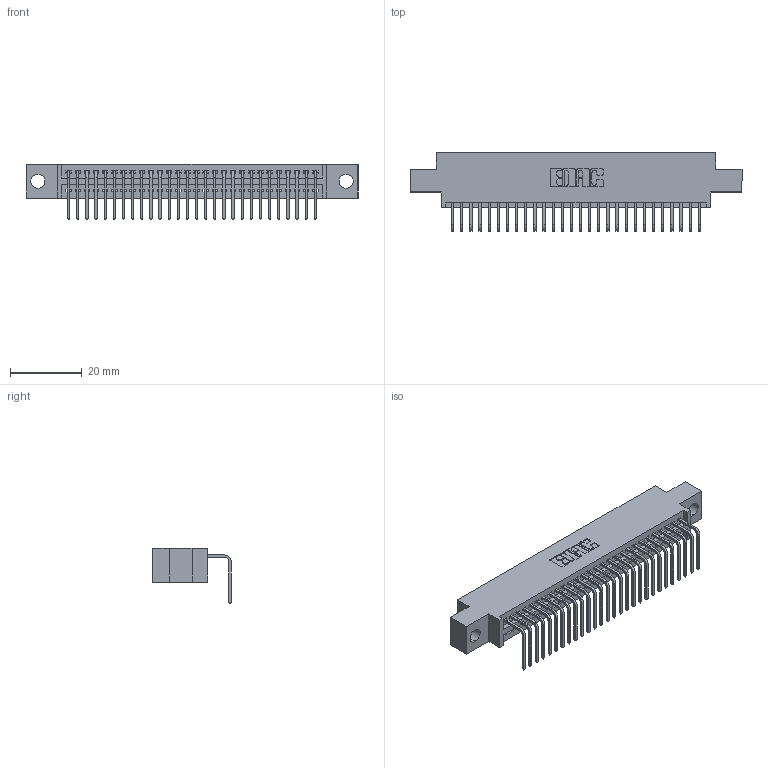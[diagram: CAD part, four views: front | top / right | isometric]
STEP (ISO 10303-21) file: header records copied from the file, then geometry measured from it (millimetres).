
FILE_DESCRIPTION (( 'STEP AP203' ), '1' );
FILE_NAME ('395-028-558-604.STEP', '2021-06-11T14:27:32', ( '' ), ( '' ), 'SwSTEP 2.0', 'SolidWorks 2020', '' );
FILE_SCHEMA (( 'CONFIG_CONTROL_DESIGN' ));
Length unit declared in the file: inch
Products named in the file (3): 345 Part_0.170 Offset - 0.156 Dia-TI; 345-292-001_558 Tail - 2; 395-028-558-604
Assembly tree (29 placements, depth 2):
  395-028-558-604
    345 Part_0.170 Offset - 0.156 Dia-TI
    345-292-001_558 Tail - 2  x28
Bounding box: 92.33 x 21.83 x 15.37 mm (x, y, z)
Volume: 8528.8 mm3; surface area: 11660.9 mm2
Topology: 29 solids, 29 shells, 1824 faces, 5485 edges, 3618 vertices
Faces by surface type: plane 1274, cylinder 550
Entity records: 23593 total; most frequent: CARTESIAN_POINT 4098, ORIENTED_EDGE 4058, DIRECTION 3597, EDGE_CURVE 2029, LINE 1785, VECTOR 1785, VERTEX_POINT 1350, AXIS2_PLACEMENT_3D 906
